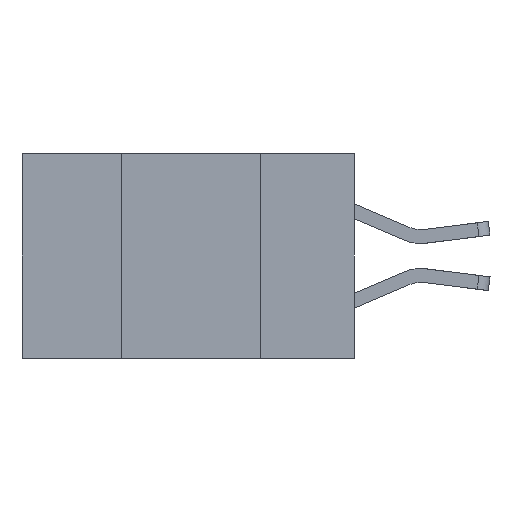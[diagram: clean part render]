
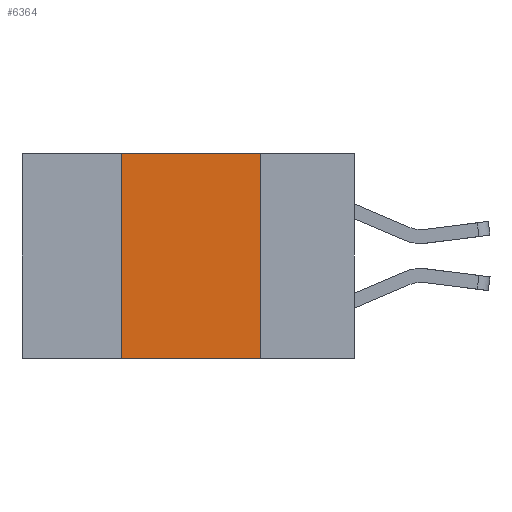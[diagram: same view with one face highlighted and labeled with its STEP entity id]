
A CAD part, left-side view. The second image highlights one B-rep face of the part: STEP entity #6364.
In plain terms, the highlighted planar face has unit normal (-1, 0, 0).
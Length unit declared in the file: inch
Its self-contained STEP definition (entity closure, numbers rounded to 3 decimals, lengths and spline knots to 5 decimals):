
#127 = ORIENTED_EDGE ( 'NONE', *, *, #754, .F. ) ;
#213 = VERTEX_POINT ( 'NONE', #5002 ) ;
#754 = EDGE_CURVE ( 'NONE', #9070, #7703, #7386, .T. ) ;
#782 = ORIENTED_EDGE ( 'NONE', *, *, #2888, .T. ) ;
#1174 = EDGE_CURVE ( 'NONE', #213, #9070, #8098, .T. ) ;
#1321 = CARTESIAN_POINT ( 'NONE',  ( 0., 0.6, 0. ) ) ;
#1352 = EDGE_LOOP ( 'NONE', ( #3499, #127, #6218, #782 ) ) ;
#2122 = EDGE_CURVE ( 'NONE', #7703, #6732, #2870, .T. ) ;
#2870 = LINE ( 'NONE', #8141, #4778 ) ;
#2888 = EDGE_CURVE ( 'NONE', #213, #6732, #3522, .T. ) ;
#3499 = ORIENTED_EDGE ( 'NONE', *, *, #2122, .F. ) ;
#3522 = LINE ( 'NONE', #5867, #9483 ) ;
#3813 = DIRECTION ( 'NONE',  ( 0., -1., 0. ) ) ;
#3830 = CARTESIAN_POINT ( 'NONE',  ( 0., 0.42, -0.37 ) ) ;
#4400 = CARTESIAN_POINT ( 'NONE',  ( 0., 0.17, 0. ) ) ;
#4532 = AXIS2_PLACEMENT_3D ( 'NONE', #9138, #9912, #5276 ) ;
#4664 = CARTESIAN_POINT ( 'NONE',  ( 0., 0.42, 0. ) ) ;
#4778 = VECTOR ( 'NONE', #8081, 39.37008 ) ;
#5002 = CARTESIAN_POINT ( 'NONE',  ( 0., 0.42, -0.37 ) ) ;
#5276 = DIRECTION ( 'NONE',  ( 0., 0., -1. ) ) ;
#5811 = VECTOR ( 'NONE', #6977, 39.37008 ) ;
#5812 = DIRECTION ( 'NONE',  ( 0., -1., 0. ) ) ;
#5867 = CARTESIAN_POINT ( 'NONE',  ( 0., 0.6, -0.37 ) ) ;
#6182 = FACE_OUTER_BOUND ( 'NONE', #1352, .T. ) ;
#6218 = ORIENTED_EDGE ( 'NONE', *, *, #1174, .F. ) ;
#6273 = CARTESIAN_POINT ( 'NONE',  ( 0., 0.17, -0.37 ) ) ;
#6364 = ADVANCED_FACE ( 'NONE', ( #6182 ), #8333, .F. ) ;
#6732 = VERTEX_POINT ( 'NONE', #6273 ) ;
#6977 = DIRECTION ( 'NONE',  ( 0., 0., 1. ) ) ;
#7125 = VECTOR ( 'NONE', #3813, 39.37008 ) ;
#7386 = LINE ( 'NONE', #1321, #7125 ) ;
#7703 = VERTEX_POINT ( 'NONE', #4400 ) ;
#8081 = DIRECTION ( 'NONE',  ( 0., 0., -1. ) ) ;
#8098 = LINE ( 'NONE', #3830, #5811 ) ;
#8141 = CARTESIAN_POINT ( 'NONE',  ( 0., 0.17, -0.37 ) ) ;
#8333 = PLANE ( 'NONE',  #4532 ) ;
#9070 = VERTEX_POINT ( 'NONE', #4664 ) ;
#9138 = CARTESIAN_POINT ( 'NONE',  ( 0., 0.6, 0. ) ) ;
#9483 = VECTOR ( 'NONE', #5812, 39.37008 ) ;
#9912 = DIRECTION ( 'NONE',  ( 1., 0., 0. ) ) ;
